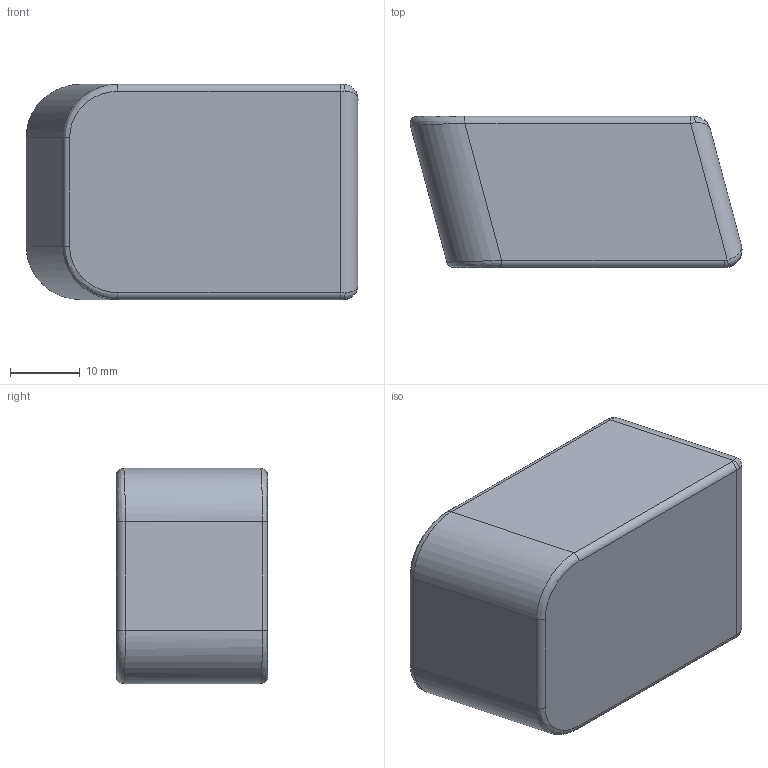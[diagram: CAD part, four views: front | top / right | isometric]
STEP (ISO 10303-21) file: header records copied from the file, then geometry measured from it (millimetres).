
FILE_DESCRIPTION(/* description */ (''),/* implementation_level */ '2;1');
FILE_NAME(/* name */ 'Menendez Mag Extended Baseplate v2.step',/* time_stamp */ '2019-08-25T22:27:39-04:00',/* author */ (''),/* organization */ (''),/* preprocessor_version */ 'ST-DEVELOPER v18',/* originating_system */ 'Autodesk Translation Framework v8.6.0.1094',/* authorisation */ '');
FILE_SCHEMA (('AUTOMOTIVE_DESIGN { 1 0 10303 214 3 1 1 }'));
Length unit declared in the file: millimetre
Products named in the file (1): Menendez Mag Extended Baseplate
Bounding box: 47.48 x 21.6 x 30.78 mm (x, y, z)
Volume: 13524.1 mm3; surface area: 7646.8 mm2
Topology: 1 solids, 1 shells, 71 faces, 184 edges, 112 vertices
Faces by surface type: plane 33, cylinder 24, bspline 10, torus 4
Entity records: 2440 total; most frequent: CARTESIAN_POINT 658, DIRECTION 366, ORIENTED_EDGE 360, EDGE_CURVE 180, AXIS2_PLACEMENT_3D 126, LINE 114, VECTOR 114, VERTEX_POINT 112
